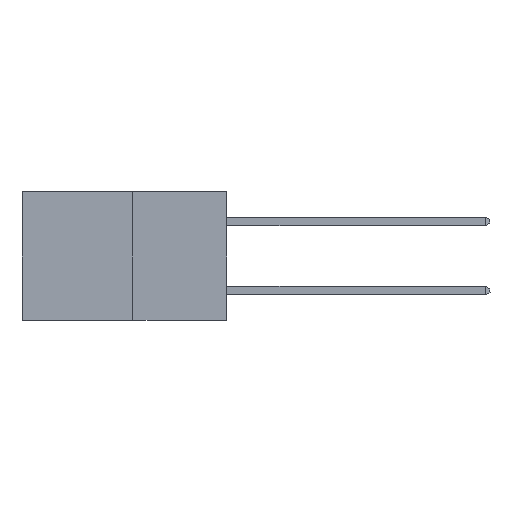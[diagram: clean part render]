
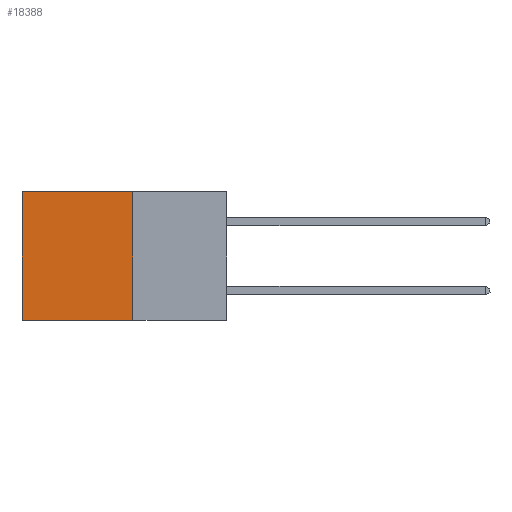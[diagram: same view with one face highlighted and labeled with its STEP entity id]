
A CAD part, left-side view. The second image highlights one B-rep face of the part: STEP entity #18388.
In plain terms, the highlighted planar face has unit normal (-1, 0, 0).
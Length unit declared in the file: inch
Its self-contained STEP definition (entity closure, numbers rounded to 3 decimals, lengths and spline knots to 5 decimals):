
#947 = LINE ( 'NONE', #9870, #21177 ) ;
#1282 = EDGE_CURVE ( 'NONE', #21370, #17171, #947, .T. ) ;
#2507 = CARTESIAN_POINT ( 'NONE',  ( 0.277, 0.27, -0.37 ) ) ;
#3719 = DIRECTION ( 'NONE',  ( 0., 0., -1. ) ) ;
#5332 = VECTOR ( 'NONE', #7362, 39.37008 ) ;
#5542 = CARTESIAN_POINT ( 'NONE',  ( 0.277, 0.27, 0. ) ) ;
#5610 = CARTESIAN_POINT ( 'NONE',  ( 0.277, 0.27, -0.37 ) ) ;
#6865 = VECTOR ( 'NONE', #14527, 39.37008 ) ;
#7362 = DIRECTION ( 'NONE',  ( 0., 1., 0. ) ) ;
#7373 = VERTEX_POINT ( 'NONE', #24023 ) ;
#7586 = PLANE ( 'NONE',  #12591 ) ;
#8080 = VERTEX_POINT ( 'NONE', #2507 ) ;
#9133 = CARTESIAN_POINT ( 'NONE',  ( 0.277, 0.59, -0.37 ) ) ;
#9800 = ORIENTED_EDGE ( 'NONE', *, *, #16996, .T. ) ;
#9870 = CARTESIAN_POINT ( 'NONE',  ( 0.277, 0.27, 0. ) ) ;
#10505 = ORIENTED_EDGE ( 'NONE', *, *, #17518, .F. ) ;
#10541 = LINE ( 'NONE', #11203, #5332 ) ;
#11189 = ORIENTED_EDGE ( 'NONE', *, *, #1282, .T. ) ;
#11203 = CARTESIAN_POINT ( 'NONE',  ( 0.277, 0.27, -0.37 ) ) ;
#12591 = AXIS2_PLACEMENT_3D ( 'NONE', #5610, #15450, #3719 ) ;
#13564 = VECTOR ( 'NONE', #15053, 39.37008 ) ;
#14527 = DIRECTION ( 'NONE',  ( 0., 0., -1. ) ) ;
#15053 = DIRECTION ( 'NONE',  ( 0., 0., -1. ) ) ;
#15450 = DIRECTION ( 'NONE',  ( 1., 0., 0. ) ) ;
#15598 = EDGE_LOOP ( 'NONE', ( #9800, #21792, #10505, #11189 ) ) ;
#16996 = EDGE_CURVE ( 'NONE', #17171, #7373, #18767, .T. ) ;
#17171 = VERTEX_POINT ( 'NONE', #21277 ) ;
#17518 = EDGE_CURVE ( 'NONE', #21370, #8080, #22470, .T. ) ;
#18388 = ADVANCED_FACE ( 'NONE', ( #19035 ), #7586, .F. ) ;
#18767 = LINE ( 'NONE', #9133, #13564 ) ;
#19035 = FACE_OUTER_BOUND ( 'NONE', #15598, .T. ) ;
#21177 = VECTOR ( 'NONE', #24378, 39.37008 ) ;
#21277 = CARTESIAN_POINT ( 'NONE',  ( 0.277, 0.59, 0. ) ) ;
#21370 = VERTEX_POINT ( 'NONE', #5542 ) ;
#21792 = ORIENTED_EDGE ( 'NONE', *, *, #23347, .F. ) ;
#22470 = LINE ( 'NONE', #24262, #6865 ) ;
#23347 = EDGE_CURVE ( 'NONE', #8080, #7373, #10541, .T. ) ;
#24023 = CARTESIAN_POINT ( 'NONE',  ( 0.277, 0.59, -0.37 ) ) ;
#24262 = CARTESIAN_POINT ( 'NONE',  ( 0.277, 0.27, -0.37 ) ) ;
#24378 = DIRECTION ( 'NONE',  ( 0., 1., 0. ) ) ;
